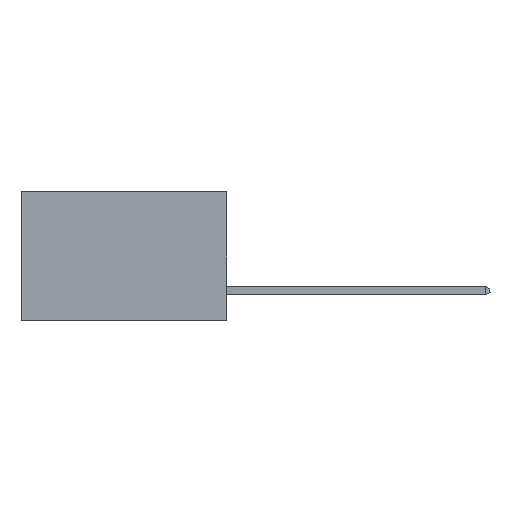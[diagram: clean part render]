
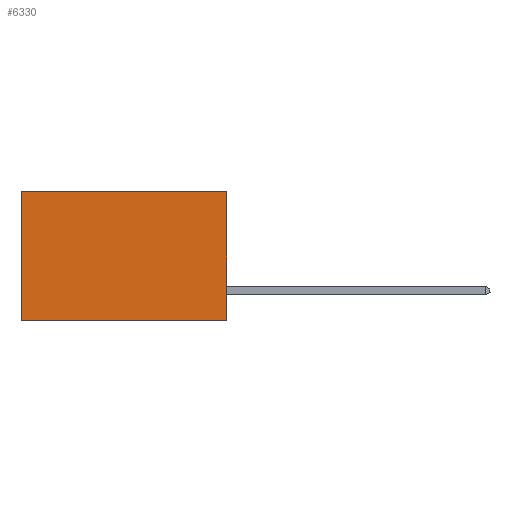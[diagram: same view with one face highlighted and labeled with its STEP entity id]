
A CAD part, left-side view. The second image highlights one B-rep face of the part: STEP entity #6330.
In plain terms, the highlighted planar face has unit normal (-1, 0, 0).
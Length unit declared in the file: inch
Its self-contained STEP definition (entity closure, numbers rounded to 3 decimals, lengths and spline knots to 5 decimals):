
#1809 = CARTESIAN_POINT ( 'NONE',  ( 0.277, 0., 0. ) ) ;
#2331 = DIRECTION ( 'NONE',  ( 0., 0., -1. ) ) ;
#4730 = LINE ( 'NONE', #17047, #14849 ) ;
#4927 = ORIENTED_EDGE ( 'NONE', *, *, #17339, .T. ) ;
#4956 = LINE ( 'NONE', #13534, #16375 ) ;
#4990 = FACE_OUTER_BOUND ( 'NONE', #19060, .T. ) ;
#5528 = VERTEX_POINT ( 'NONE', #25513 ) ;
#5700 = DIRECTION ( 'NONE',  ( 0., 0., -1. ) ) ;
#5748 = DIRECTION ( 'NONE',  ( 1., 0., 0. ) ) ;
#5779 = CARTESIAN_POINT ( 'NONE',  ( 0.277, 0., -0.37 ) ) ;
#5867 = PLANE ( 'NONE',  #11994 ) ;
#6330 = ADVANCED_FACE ( 'NONE', ( #4990 ), #5867, .F. ) ;
#6956 = DIRECTION ( 'NONE',  ( 0., 1., 0. ) ) ;
#7488 = DIRECTION ( 'NONE',  ( 0., 1., 0. ) ) ;
#8246 = VECTOR ( 'NONE', #7488, 39.37008 ) ;
#8397 = CARTESIAN_POINT ( 'NONE',  ( 0.277, 0., -0.37 ) ) ;
#10296 = ORIENTED_EDGE ( 'NONE', *, *, #12181, .F. ) ;
#10889 = ORIENTED_EDGE ( 'NONE', *, *, #23370, .F. ) ;
#11275 = CARTESIAN_POINT ( 'NONE',  ( 0.277, 0.59, -0.37 ) ) ;
#11994 = AXIS2_PLACEMENT_3D ( 'NONE', #5779, #5748, #5700 ) ;
#12181 = EDGE_CURVE ( 'NONE', #16768, #20940, #13311, .T. ) ;
#12669 = VECTOR ( 'NONE', #2331, 39.37008 ) ;
#13311 = LINE ( 'NONE', #8397, #12669 ) ;
#13534 = CARTESIAN_POINT ( 'NONE',  ( 0.277, 0.59, -0.37 ) ) ;
#13604 = CARTESIAN_POINT ( 'NONE',  ( 0.277, 0., -0.37 ) ) ;
#14849 = VECTOR ( 'NONE', #6956, 39.37008 ) ;
#15587 = DIRECTION ( 'NONE',  ( 0., 0., -1. ) ) ;
#15624 = CARTESIAN_POINT ( 'NONE',  ( 0.277, 0., 0. ) ) ;
#16375 = VECTOR ( 'NONE', #15587, 39.37008 ) ;
#16768 = VERTEX_POINT ( 'NONE', #1809 ) ;
#17047 = CARTESIAN_POINT ( 'NONE',  ( 0.277, 0., -0.37 ) ) ;
#17339 = EDGE_CURVE ( 'NONE', #5528, #21391, #4956, .T. ) ;
#19060 = EDGE_LOOP ( 'NONE', ( #4927, #10889, #10296, #20920 ) ) ;
#20920 = ORIENTED_EDGE ( 'NONE', *, *, #21510, .T. ) ;
#20940 = VERTEX_POINT ( 'NONE', #13604 ) ;
#21391 = VERTEX_POINT ( 'NONE', #11275 ) ;
#21510 = EDGE_CURVE ( 'NONE', #16768, #5528, #24482, .T. ) ;
#23370 = EDGE_CURVE ( 'NONE', #20940, #21391, #4730, .T. ) ;
#24482 = LINE ( 'NONE', #15624, #8246 ) ;
#25513 = CARTESIAN_POINT ( 'NONE',  ( 0.277, 0.59, 0. ) ) ;
